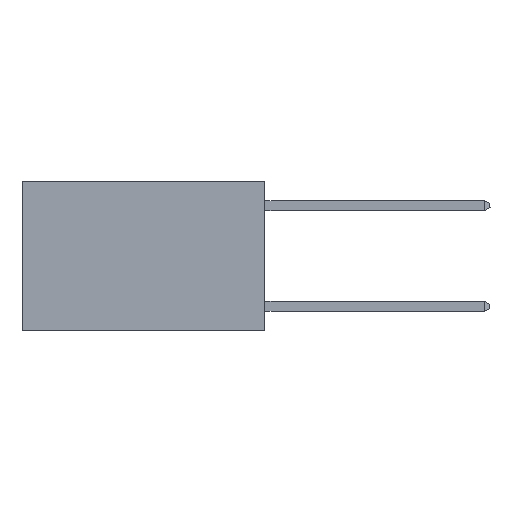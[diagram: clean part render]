
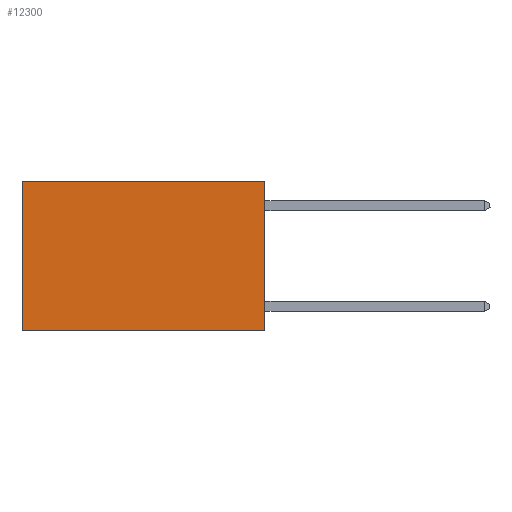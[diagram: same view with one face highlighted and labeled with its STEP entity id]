
A CAD part, left-side view. The second image highlights one B-rep face of the part: STEP entity #12300.
In plain terms, the highlighted planar face has unit normal (-1, 0, 0).
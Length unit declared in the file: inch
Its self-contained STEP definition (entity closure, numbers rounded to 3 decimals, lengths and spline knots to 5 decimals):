
#266 = AXIS2_PLACEMENT_3D ( 'NONE', #11362, #6884, #14449 ) ;
#333 = DIRECTION ( 'NONE',  ( 0., 1., 0. ) ) ;
#1097 = VERTEX_POINT ( 'NONE', #6953 ) ;
#1484 = LINE ( 'NONE', #3800, #6883 ) ;
#1648 = CARTESIAN_POINT ( 'NONE',  ( 0.2625, 0., 0. ) ) ;
#1806 = VECTOR ( 'NONE', #10977, 39.37008 ) ;
#1975 = EDGE_LOOP ( 'NONE', ( #12588, #6878, #9868, #7226 ) ) ;
#2120 = FACE_OUTER_BOUND ( 'NONE', #1975, .T. ) ;
#2287 = VECTOR ( 'NONE', #4252, 39.37008 ) ;
#3024 = VERTEX_POINT ( 'NONE', #12433 ) ;
#3498 = VERTEX_POINT ( 'NONE', #1648 ) ;
#3619 = EDGE_CURVE ( 'NONE', #3498, #4963, #5356, .T. ) ;
#3800 = CARTESIAN_POINT ( 'NONE',  ( 0.2625, 0., -0.37 ) ) ;
#3982 = CARTESIAN_POINT ( 'NONE',  ( 0.2625, 0., 0. ) ) ;
#4252 = DIRECTION ( 'NONE',  ( 0., 0., -1. ) ) ;
#4963 = VERTEX_POINT ( 'NONE', #14003 ) ;
#5290 = CARTESIAN_POINT ( 'NONE',  ( 0.2625, 0.6, 0. ) ) ;
#5320 = CARTESIAN_POINT ( 'NONE',  ( 0.2625, 0., 0. ) ) ;
#5356 = LINE ( 'NONE', #3982, #2287 ) ;
#5727 = PLANE ( 'NONE',  #266 ) ;
#6435 = DIRECTION ( 'NONE',  ( 0., 0., -1. ) ) ;
#6878 = ORIENTED_EDGE ( 'NONE', *, *, #9541, .F. ) ;
#6883 = VECTOR ( 'NONE', #333, 39.37008 ) ;
#6884 = DIRECTION ( 'NONE',  ( 1., 0., 0. ) ) ;
#6953 = CARTESIAN_POINT ( 'NONE',  ( 0.2625, 0.6, -0.37 ) ) ;
#7226 = ORIENTED_EDGE ( 'NONE', *, *, #10637, .T. ) ;
#7876 = VECTOR ( 'NONE', #6435, 39.37008 ) ;
#8487 = EDGE_CURVE ( 'NONE', #3024, #1097, #10544, .T. ) ;
#9541 = EDGE_CURVE ( 'NONE', #4963, #1097, #1484, .T. ) ;
#9868 = ORIENTED_EDGE ( 'NONE', *, *, #3619, .F. ) ;
#10544 = LINE ( 'NONE', #5290, #7876 ) ;
#10637 = EDGE_CURVE ( 'NONE', #3498, #3024, #10933, .T. ) ;
#10933 = LINE ( 'NONE', #5320, #1806 ) ;
#10977 = DIRECTION ( 'NONE',  ( 0., 1., 0. ) ) ;
#11362 = CARTESIAN_POINT ( 'NONE',  ( 0.2625, 0., 0. ) ) ;
#12300 = ADVANCED_FACE ( 'NONE', ( #2120 ), #5727, .F. ) ;
#12433 = CARTESIAN_POINT ( 'NONE',  ( 0.2625, 0.6, 0. ) ) ;
#12588 = ORIENTED_EDGE ( 'NONE', *, *, #8487, .T. ) ;
#14003 = CARTESIAN_POINT ( 'NONE',  ( 0.2625, 0., -0.37 ) ) ;
#14449 = DIRECTION ( 'NONE',  ( 0., 0., -1. ) ) ;
